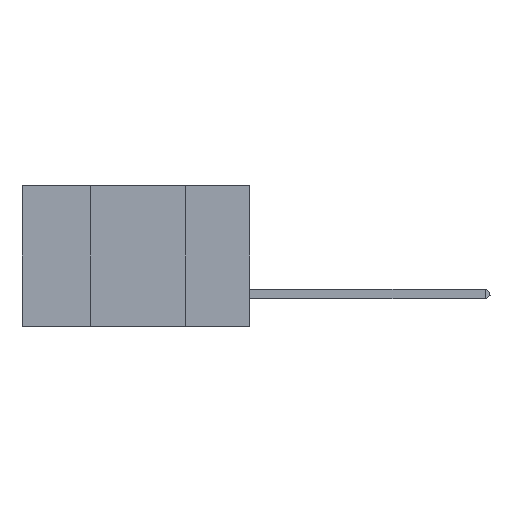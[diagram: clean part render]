
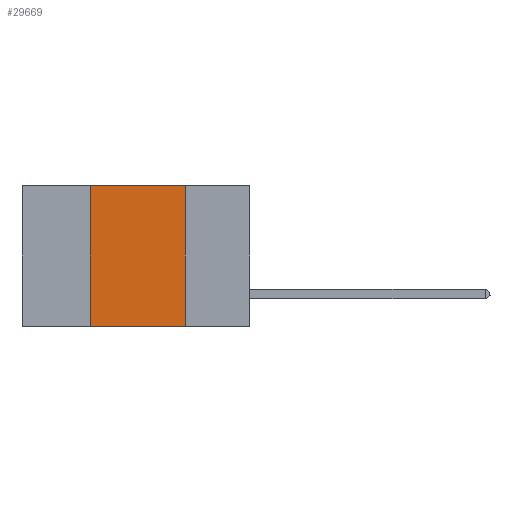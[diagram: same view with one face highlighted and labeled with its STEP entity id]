
A CAD part, left-side view. The second image highlights one B-rep face of the part: STEP entity #29669.
In plain terms, the highlighted planar face has unit normal (-1, 0, 0).
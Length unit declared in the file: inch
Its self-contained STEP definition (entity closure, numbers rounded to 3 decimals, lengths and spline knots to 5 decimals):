
#168 = VERTEX_POINT ( 'NONE', #26061 ) ;
#741 = VECTOR ( 'NONE', #16417, 39.37008 ) ;
#1290 = CARTESIAN_POINT ( 'NONE',  ( 0., 0.42, 0. ) ) ;
#1825 = ORIENTED_EDGE ( 'NONE', *, *, #6700, .F. ) ;
#2558 = CARTESIAN_POINT ( 'NONE',  ( 0., 0.6, -0.37 ) ) ;
#3879 = EDGE_CURVE ( 'NONE', #9826, #168, #14270, .T. ) ;
#5960 = FACE_OUTER_BOUND ( 'NONE', #14918, .T. ) ;
#6700 = EDGE_CURVE ( 'NONE', #168, #39857, #31161, .T. ) ;
#8116 = ORIENTED_EDGE ( 'NONE', *, *, #40683, .F. ) ;
#9826 = VERTEX_POINT ( 'NONE', #35013 ) ;
#10333 = ORIENTED_EDGE ( 'NONE', *, *, #3879, .F. ) ;
#13004 = DIRECTION ( 'NONE',  ( 1., 0., 0. ) ) ;
#13833 = LINE ( 'NONE', #1290, #44521 ) ;
#14270 = LINE ( 'NONE', #39690, #41150 ) ;
#14918 = EDGE_LOOP ( 'NONE', ( #1825, #10333, #8116, #33638 ) ) ;
#16417 = DIRECTION ( 'NONE',  ( 0., -1., 0. ) ) ;
#18689 = DIRECTION ( 'NONE',  ( 0., 0., 1. ) ) ;
#25026 = CARTESIAN_POINT ( 'NONE',  ( 0., 0.17, -0.37 ) ) ;
#25853 = DIRECTION ( 'NONE',  ( 0., 0., -1. ) ) ;
#26061 = CARTESIAN_POINT ( 'NONE',  ( 0., 0.17, 0. ) ) ;
#29669 = ADVANCED_FACE ( 'NONE', ( #5960 ), #44379, .F. ) ;
#30025 = CARTESIAN_POINT ( 'NONE',  ( 0., 0.6, 0. ) ) ;
#31161 = LINE ( 'NONE', #39740, #44840 ) ;
#32003 = EDGE_CURVE ( 'NONE', #38867, #39857, #38458, .T. ) ;
#32724 = CARTESIAN_POINT ( 'NONE',  ( 0., 0.42, -0.37 ) ) ;
#33527 = DIRECTION ( 'NONE',  ( 0., 0., -1. ) ) ;
#33638 = ORIENTED_EDGE ( 'NONE', *, *, #32003, .T. ) ;
#35013 = CARTESIAN_POINT ( 'NONE',  ( 0., 0.42, 0. ) ) ;
#38458 = LINE ( 'NONE', #2558, #741 ) ;
#38867 = VERTEX_POINT ( 'NONE', #32724 ) ;
#39690 = CARTESIAN_POINT ( 'NONE',  ( 0., 0.6, 0. ) ) ;
#39740 = CARTESIAN_POINT ( 'NONE',  ( 0., 0.17, 0. ) ) ;
#39857 = VERTEX_POINT ( 'NONE', #25026 ) ;
#40683 = EDGE_CURVE ( 'NONE', #38867, #9826, #13833, .T. ) ;
#41150 = VECTOR ( 'NONE', #43906, 39.37008 ) ;
#43906 = DIRECTION ( 'NONE',  ( 0., -1., 0. ) ) ;
#44379 = PLANE ( 'NONE',  #44746 ) ;
#44521 = VECTOR ( 'NONE', #18689, 39.37008 ) ;
#44746 = AXIS2_PLACEMENT_3D ( 'NONE', #30025, #13004, #33527 ) ;
#44840 = VECTOR ( 'NONE', #25853, 39.37008 ) ;
